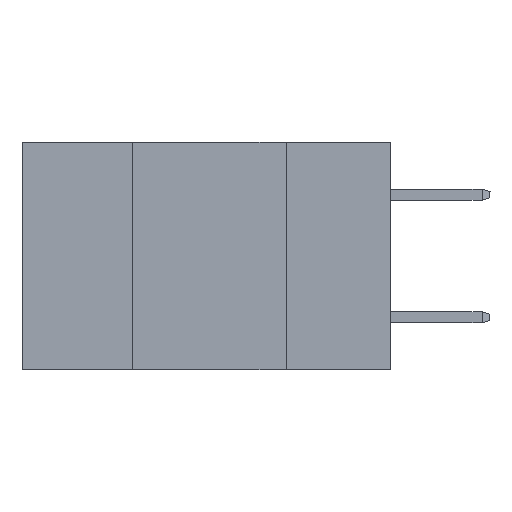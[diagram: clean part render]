
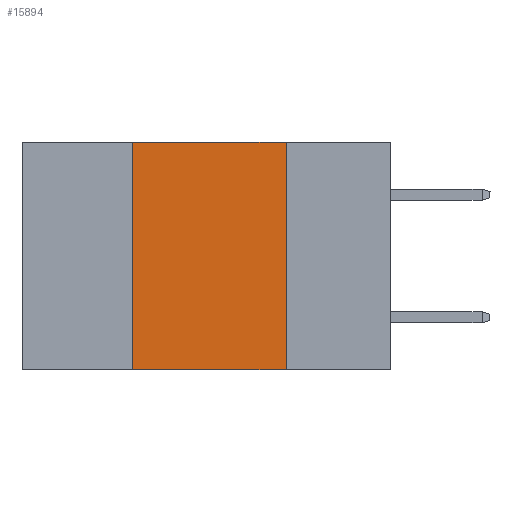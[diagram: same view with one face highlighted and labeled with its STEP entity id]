
A CAD part, left-side view. The second image highlights one B-rep face of the part: STEP entity #15894.
In plain terms, the highlighted planar face has unit normal (-1, 0, 0).
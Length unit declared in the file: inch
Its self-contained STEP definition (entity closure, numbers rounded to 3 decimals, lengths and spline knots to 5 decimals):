
#441 = EDGE_CURVE ( 'NONE', #15257, #12123, #2810, .T. ) ;
#1716 = ORIENTED_EDGE ( 'NONE', *, *, #441, .F. ) ;
#1988 = PLANE ( 'NONE',  #20084 ) ;
#2434 = CARTESIAN_POINT ( 'NONE',  ( 0., 0.17, -0.37 ) ) ;
#2810 = LINE ( 'NONE', #6094, #8024 ) ;
#2986 = VERTEX_POINT ( 'NONE', #2434 ) ;
#5023 = ORIENTED_EDGE ( 'NONE', *, *, #13749, .T. ) ;
#5203 = VERTEX_POINT ( 'NONE', #17613 ) ;
#5255 = VECTOR ( 'NONE', #21374, 39.37008 ) ;
#5727 = CARTESIAN_POINT ( 'NONE',  ( 0., 0.6, 0. ) ) ;
#5980 = EDGE_CURVE ( 'NONE', #12123, #5203, #19639, .T. ) ;
#6094 = CARTESIAN_POINT ( 'NONE',  ( 0., 0.42, 0. ) ) ;
#7314 = ORIENTED_EDGE ( 'NONE', *, *, #5980, .F. ) ;
#8024 = VECTOR ( 'NONE', #15145, 39.37008 ) ;
#8633 = DIRECTION ( 'NONE',  ( 0., -1., 0. ) ) ;
#8816 = CARTESIAN_POINT ( 'NONE',  ( 0., 0.17, 0. ) ) ;
#10918 = LINE ( 'NONE', #8816, #11201 ) ;
#11201 = VECTOR ( 'NONE', #18171, 39.37008 ) ;
#12123 = VERTEX_POINT ( 'NONE', #16695 ) ;
#12583 = ORIENTED_EDGE ( 'NONE', *, *, #20601, .F. ) ;
#13062 = DIRECTION ( 'NONE',  ( 0., 0., -1. ) ) ;
#13749 = EDGE_CURVE ( 'NONE', #15257, #2986, #14122, .T. ) ;
#14122 = LINE ( 'NONE', #23025, #5255 ) ;
#15145 = DIRECTION ( 'NONE',  ( 0., 0., 1. ) ) ;
#15257 = VERTEX_POINT ( 'NONE', #22558 ) ;
#15894 = ADVANCED_FACE ( 'NONE', ( #22745 ), #1988, .F. ) ;
#16695 = CARTESIAN_POINT ( 'NONE',  ( 0., 0.42, 0. ) ) ;
#17613 = CARTESIAN_POINT ( 'NONE',  ( 0., 0.17, 0. ) ) ;
#18171 = DIRECTION ( 'NONE',  ( 0., 0., -1. ) ) ;
#18623 = DIRECTION ( 'NONE',  ( 1., 0., 0. ) ) ;
#19545 = CARTESIAN_POINT ( 'NONE',  ( 0., 0.6, 0. ) ) ;
#19639 = LINE ( 'NONE', #19545, #22607 ) ;
#20084 = AXIS2_PLACEMENT_3D ( 'NONE', #5727, #18623, #13062 ) ;
#20601 = EDGE_CURVE ( 'NONE', #5203, #2986, #10918, .T. ) ;
#21374 = DIRECTION ( 'NONE',  ( 0., -1., 0. ) ) ;
#22558 = CARTESIAN_POINT ( 'NONE',  ( 0., 0.42, -0.37 ) ) ;
#22607 = VECTOR ( 'NONE', #8633, 39.37008 ) ;
#22745 = FACE_OUTER_BOUND ( 'NONE', #22882, .T. ) ;
#22882 = EDGE_LOOP ( 'NONE', ( #12583, #7314, #1716, #5023 ) ) ;
#23025 = CARTESIAN_POINT ( 'NONE',  ( 0., 0.6, -0.37 ) ) ;
